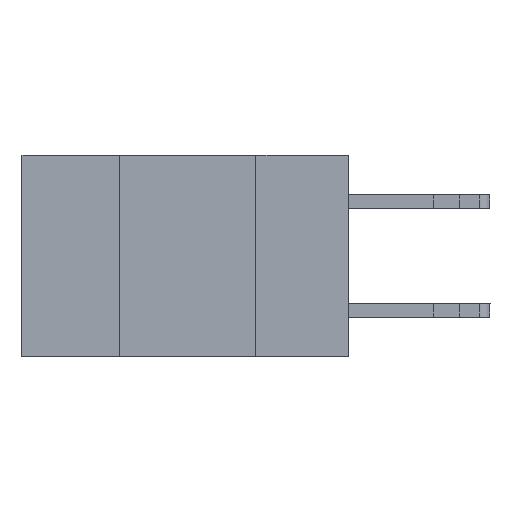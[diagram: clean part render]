
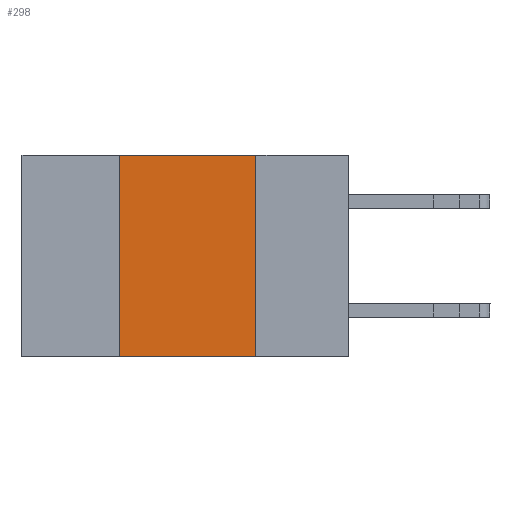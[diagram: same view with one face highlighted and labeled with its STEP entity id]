
A CAD part, left-side view. The second image highlights one B-rep face of the part: STEP entity #298.
In plain terms, the highlighted planar face has unit normal (-1, 0, 0).
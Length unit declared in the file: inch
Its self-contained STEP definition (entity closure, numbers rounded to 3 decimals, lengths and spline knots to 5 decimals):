
#298 = ADVANCED_FACE ( 'NONE', ( #2167 ), #14088, .F. ) ;
#564 = CARTESIAN_POINT ( 'NONE',  ( 0., 0.6, 0. ) ) ;
#1099 = DIRECTION ( 'NONE',  ( 1., 0., 0. ) ) ;
#1115 = CARTESIAN_POINT ( 'NONE',  ( 0., 0.17, -0.37 ) ) ;
#1296 = EDGE_LOOP ( 'NONE', ( #2932, #20033, #15077, #7946 ) ) ;
#1865 = LINE ( 'NONE', #3998, #9714 ) ;
#2167 = FACE_OUTER_BOUND ( 'NONE', #1296, .T. ) ;
#2497 = VERTEX_POINT ( 'NONE', #21229 ) ;
#2738 = DIRECTION ( 'NONE',  ( 0., -1., 0. ) ) ;
#2932 = ORIENTED_EDGE ( 'NONE', *, *, #14394, .F. ) ;
#3802 = DIRECTION ( 'NONE',  ( 0., 0., -1. ) ) ;
#3974 = VERTEX_POINT ( 'NONE', #25783 ) ;
#3998 = CARTESIAN_POINT ( 'NONE',  ( 0., 0.17, 0. ) ) ;
#5574 = VECTOR ( 'NONE', #23611, 39.37008 ) ;
#5617 = CARTESIAN_POINT ( 'NONE',  ( 0., 0.6, -0.37 ) ) ;
#6850 = VECTOR ( 'NONE', #2738, 39.37008 ) ;
#7946 = ORIENTED_EDGE ( 'NONE', *, *, #27887, .T. ) ;
#9182 = CARTESIAN_POINT ( 'NONE',  ( 0., 0.17, 0. ) ) ;
#9246 = LINE ( 'NONE', #5617, #20713 ) ;
#9714 = VECTOR ( 'NONE', #3802, 39.37008 ) ;
#10421 = VERTEX_POINT ( 'NONE', #1115 ) ;
#11226 = EDGE_CURVE ( 'NONE', #3974, #16038, #26449, .T. ) ;
#12958 = CARTESIAN_POINT ( 'NONE',  ( 0., 0.42, 0. ) ) ;
#14088 = PLANE ( 'NONE',  #25053 ) ;
#14394 = EDGE_CURVE ( 'NONE', #16038, #10421, #1865, .T. ) ;
#15077 = ORIENTED_EDGE ( 'NONE', *, *, #15901, .F. ) ;
#15376 = LINE ( 'NONE', #12958, #5574 ) ;
#15901 = EDGE_CURVE ( 'NONE', #2497, #3974, #15376, .T. ) ;
#16038 = VERTEX_POINT ( 'NONE', #9182 ) ;
#18235 = DIRECTION ( 'NONE',  ( 0., 0., -1. ) ) ;
#20033 = ORIENTED_EDGE ( 'NONE', *, *, #11226, .F. ) ;
#20691 = CARTESIAN_POINT ( 'NONE',  ( 0., 0.6, 0. ) ) ;
#20713 = VECTOR ( 'NONE', #21301, 39.37008 ) ;
#21229 = CARTESIAN_POINT ( 'NONE',  ( 0., 0.42, -0.37 ) ) ;
#21301 = DIRECTION ( 'NONE',  ( 0., -1., 0. ) ) ;
#23611 = DIRECTION ( 'NONE',  ( 0., 0., 1. ) ) ;
#25053 = AXIS2_PLACEMENT_3D ( 'NONE', #20691, #1099, #18235 ) ;
#25783 = CARTESIAN_POINT ( 'NONE',  ( 0., 0.42, 0. ) ) ;
#26449 = LINE ( 'NONE', #564, #6850 ) ;
#27887 = EDGE_CURVE ( 'NONE', #2497, #10421, #9246, .T. ) ;
